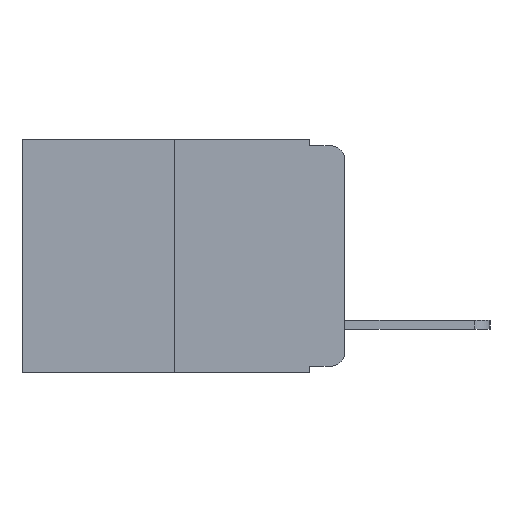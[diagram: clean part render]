
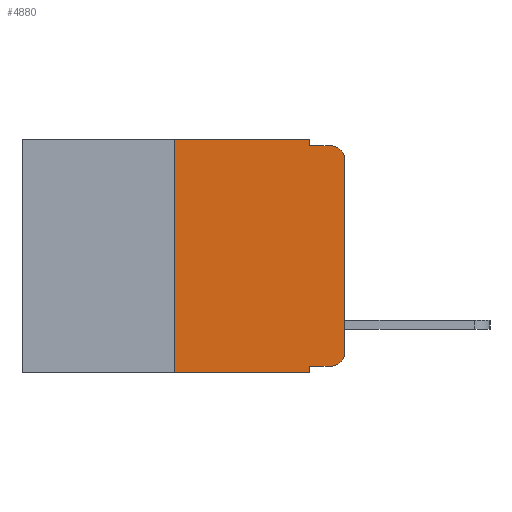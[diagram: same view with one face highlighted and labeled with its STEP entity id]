
A CAD part, left-side view. The second image highlights one B-rep face of the part: STEP entity #4880.
In plain terms, the highlighted planar face has unit normal (-1, 0, 0).
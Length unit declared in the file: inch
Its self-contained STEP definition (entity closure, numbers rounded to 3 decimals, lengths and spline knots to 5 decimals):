
#39 = ORIENTED_EDGE ( 'NONE', *, *, #15111, .T. ) ;
#148 = EDGE_CURVE ( 'NONE', #11275, #15754, #9049, .T. ) ;
#205 = DIRECTION ( 'NONE',  ( -1., 0., 0. ) ) ;
#561 = CARTESIAN_POINT ( 'NONE',  ( 0., 0.473, -0.343 ) ) ;
#728 = CARTESIAN_POINT ( 'NONE',  ( 0., 0.051, 0. ) ) ;
#934 = AXIS2_PLACEMENT_3D ( 'NONE', #13185, #15646, #15548 ) ;
#1034 = ORIENTED_EDGE ( 'NONE', *, *, #148, .F. ) ;
#1186 = EDGE_CURVE ( 'NONE', #5107, #3644, #2754, .T. ) ;
#1194 = VECTOR ( 'NONE', #16676, 39.37008 ) ;
#1448 = VECTOR ( 'NONE', #10963, 39.37008 ) ;
#1818 = VECTOR ( 'NONE', #9047, 39.37008 ) ;
#2145 = EDGE_CURVE ( 'NONE', #12877, #8779, #9422, .T. ) ;
#2147 = CIRCLE ( 'NONE', #14668, 0.02 ) ;
#2405 = DIRECTION ( 'NONE',  ( 0., 0., -1. ) ) ;
#2754 = LINE ( 'NONE', #15201, #13535 ) ;
#2933 = DIRECTION ( 'NONE',  ( -1., 0., 0. ) ) ;
#3003 = EDGE_CURVE ( 'NONE', #3644, #11275, #15037, .T. ) ;
#3070 = CARTESIAN_POINT ( 'NONE',  ( 0., 0.02, -0.313 ) ) ;
#3128 = EDGE_CURVE ( 'NONE', #12877, #11217, #6755, .T. ) ;
#3644 = VERTEX_POINT ( 'NONE', #5297 ) ;
#3733 = CARTESIAN_POINT ( 'NONE',  ( 0., 0., -0.313 ) ) ;
#4102 = EDGE_CURVE ( 'NONE', #11217, #16757, #2147, .T. ) ;
#4152 = DIRECTION ( 'NONE',  ( 0., -1., 0. ) ) ;
#4210 = ORIENTED_EDGE ( 'NONE', *, *, #3128, .T. ) ;
#4354 = DIRECTION ( 'NONE',  ( 0., -1., 0. ) ) ;
#4413 = CARTESIAN_POINT ( 'NONE',  ( 0., 0.051, 0. ) ) ;
#4769 = EDGE_CURVE ( 'NONE', #5107, #8779, #9277, .T. ) ;
#4823 = ORIENTED_EDGE ( 'NONE', *, *, #3003, .F. ) ;
#4829 = DIRECTION ( 'NONE',  ( 0., 0., -1. ) ) ;
#4857 = VECTOR ( 'NONE', #4152, 39.37008 ) ;
#4880 = ADVANCED_FACE ( 'NONE', ( #17026 ), #16251, .F. ) ;
#4973 = CARTESIAN_POINT ( 'NONE',  ( 0., 0.02, -0.01 ) ) ;
#4980 = CARTESIAN_POINT ( 'NONE',  ( 0., 0.051, -0.333 ) ) ;
#4983 = LINE ( 'NONE', #13863, #14758 ) ;
#5107 = VERTEX_POINT ( 'NONE', #10169 ) ;
#5297 = CARTESIAN_POINT ( 'NONE',  ( 0., 0.25, 0. ) ) ;
#5623 = CARTESIAN_POINT ( 'NONE',  ( 0., 0.051, 0. ) ) ;
#5710 = CARTESIAN_POINT ( 'NONE',  ( 0., 0.051, -0.343 ) ) ;
#5739 = VERTEX_POINT ( 'NONE', #14353 ) ;
#6755 = LINE ( 'NONE', #4980, #16718 ) ;
#7379 = AXIS2_PLACEMENT_3D ( 'NONE', #8657, #205, #10033 ) ;
#8657 = CARTESIAN_POINT ( 'NONE',  ( 0., 0.02, -0.03 ) ) ;
#8779 = VERTEX_POINT ( 'NONE', #5710 ) ;
#9047 = DIRECTION ( 'NONE',  ( 0., -1., 0. ) ) ;
#9049 = LINE ( 'NONE', #5623, #1194 ) ;
#9124 = CARTESIAN_POINT ( 'NONE',  ( 0., 0.473, 0. ) ) ;
#9277 = LINE ( 'NONE', #561, #1448 ) ;
#9422 = LINE ( 'NONE', #4413, #12905 ) ;
#10015 = CARTESIAN_POINT ( 'NONE',  ( 0., 0.051, -0.333 ) ) ;
#10033 = DIRECTION ( 'NONE',  ( 0., 0., -1. ) ) ;
#10169 = CARTESIAN_POINT ( 'NONE',  ( 0., 0.25, -0.343 ) ) ;
#10963 = DIRECTION ( 'NONE',  ( 0., -1., 0. ) ) ;
#11217 = VERTEX_POINT ( 'NONE', #14200 ) ;
#11275 = VERTEX_POINT ( 'NONE', #728 ) ;
#11398 = ORIENTED_EDGE ( 'NONE', *, *, #4102, .T. ) ;
#11417 = DIRECTION ( 'NONE',  ( 0., 0., 1. ) ) ;
#11593 = ORIENTED_EDGE ( 'NONE', *, *, #16713, .F. ) ;
#12711 = LINE ( 'NONE', #15501, #1818 ) ;
#12877 = VERTEX_POINT ( 'NONE', #10015 ) ;
#12905 = VECTOR ( 'NONE', #4829, 39.37008 ) ;
#13044 = VERTEX_POINT ( 'NONE', #4973 ) ;
#13185 = CARTESIAN_POINT ( 'NONE',  ( 0., 0.473, 0. ) ) ;
#13215 = ORIENTED_EDGE ( 'NONE', *, *, #1186, .F. ) ;
#13535 = VECTOR ( 'NONE', #11417, 39.37008 ) ;
#13863 = CARTESIAN_POINT ( 'NONE',  ( 0., 0., 0. ) ) ;
#14200 = CARTESIAN_POINT ( 'NONE',  ( 0., 0.02, -0.333 ) ) ;
#14353 = CARTESIAN_POINT ( 'NONE',  ( 0., 0., -0.03 ) ) ;
#14611 = ORIENTED_EDGE ( 'NONE', *, *, #15915, .T. ) ;
#14668 = AXIS2_PLACEMENT_3D ( 'NONE', #3070, #2933, #2405 ) ;
#14758 = VECTOR ( 'NONE', #15115, 39.37008 ) ;
#14929 = CIRCLE ( 'NONE', #7379, 0.02 ) ;
#15037 = LINE ( 'NONE', #9124, #4857 ) ;
#15103 = EDGE_LOOP ( 'NONE', ( #39, #14611, #11593, #1034, #4823, #13215, #16525, #16884, #4210, #11398 ) ) ;
#15111 = EDGE_CURVE ( 'NONE', #16757, #5739, #4983, .T. ) ;
#15115 = DIRECTION ( 'NONE',  ( 0., 0., 1. ) ) ;
#15201 = CARTESIAN_POINT ( 'NONE',  ( 0., 0.25, 0. ) ) ;
#15501 = CARTESIAN_POINT ( 'NONE',  ( 0., 0.051, -0.01 ) ) ;
#15548 = DIRECTION ( 'NONE',  ( 0., 0., -1. ) ) ;
#15646 = DIRECTION ( 'NONE',  ( 1., 0., 0. ) ) ;
#15754 = VERTEX_POINT ( 'NONE', #17277 ) ;
#15915 = EDGE_CURVE ( 'NONE', #5739, #13044, #14929, .T. ) ;
#16251 = PLANE ( 'NONE',  #934 ) ;
#16525 = ORIENTED_EDGE ( 'NONE', *, *, #4769, .T. ) ;
#16676 = DIRECTION ( 'NONE',  ( 0., 0., -1. ) ) ;
#16713 = EDGE_CURVE ( 'NONE', #15754, #13044, #12711, .T. ) ;
#16718 = VECTOR ( 'NONE', #4354, 39.37008 ) ;
#16757 = VERTEX_POINT ( 'NONE', #3733 ) ;
#16884 = ORIENTED_EDGE ( 'NONE', *, *, #2145, .F. ) ;
#17026 = FACE_OUTER_BOUND ( 'NONE', #15103, .T. ) ;
#17277 = CARTESIAN_POINT ( 'NONE',  ( 0., 0.051, -0.01 ) ) ;
